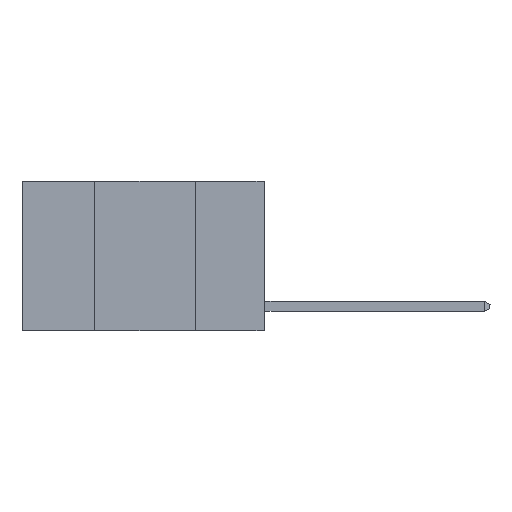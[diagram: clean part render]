
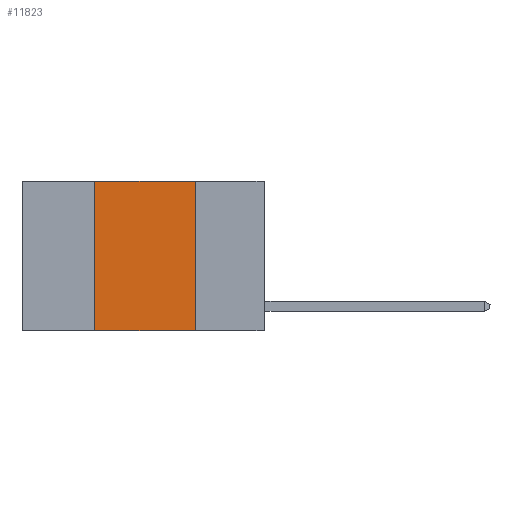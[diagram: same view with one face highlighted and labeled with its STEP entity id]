
A CAD part, left-side view. The second image highlights one B-rep face of the part: STEP entity #11823.
In plain terms, the highlighted planar face has unit normal (-1, 0, 0).
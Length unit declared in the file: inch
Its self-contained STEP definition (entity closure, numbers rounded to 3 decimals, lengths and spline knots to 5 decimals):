
#327 = VECTOR ( 'NONE', #13851, 39.37008 ) ;
#331 = CARTESIAN_POINT ( 'NONE',  ( 0., 0.6, 0. ) ) ;
#853 = LINE ( 'NONE', #331, #14843 ) ;
#2307 = VERTEX_POINT ( 'NONE', #4782 ) ;
#2994 = VERTEX_POINT ( 'NONE', #6998 ) ;
#4344 = CARTESIAN_POINT ( 'NONE',  ( 0., 0.42, 0. ) ) ;
#4782 = CARTESIAN_POINT ( 'NONE',  ( 0., 0.17, -0.37 ) ) ;
#4846 = EDGE_LOOP ( 'NONE', ( #9016, #16720, #15301, #22630 ) ) ;
#5851 = DIRECTION ( 'NONE',  ( 0., -1., 0. ) ) ;
#6039 = LINE ( 'NONE', #4344, #15748 ) ;
#6593 = CARTESIAN_POINT ( 'NONE',  ( 0., 0.6, -0.37 ) ) ;
#6890 = DIRECTION ( 'NONE',  ( 0., 0., -1. ) ) ;
#6998 = CARTESIAN_POINT ( 'NONE',  ( 0., 0.17, 0. ) ) ;
#7454 = CARTESIAN_POINT ( 'NONE',  ( 0., 0.6, 0. ) ) ;
#8240 = CARTESIAN_POINT ( 'NONE',  ( 0., 0.42, -0.37 ) ) ;
#8702 = CARTESIAN_POINT ( 'NONE',  ( 0., 0.17, 0. ) ) ;
#9016 = ORIENTED_EDGE ( 'NONE', *, *, #10426, .F. ) ;
#9424 = EDGE_CURVE ( 'NONE', #10244, #22296, #6039, .T. ) ;
#10043 = LINE ( 'NONE', #6593, #327 ) ;
#10093 = EDGE_CURVE ( 'NONE', #22296, #2994, #853, .T. ) ;
#10244 = VERTEX_POINT ( 'NONE', #8240 ) ;
#10426 = EDGE_CURVE ( 'NONE', #2994, #2307, #17103, .T. ) ;
#11143 = DIRECTION ( 'NONE',  ( 0., 0., -1. ) ) ;
#11823 = ADVANCED_FACE ( 'NONE', ( #20702 ), #12908, .F. ) ;
#12282 = VECTOR ( 'NONE', #6890, 39.37008 ) ;
#12908 = PLANE ( 'NONE',  #17434 ) ;
#12997 = CARTESIAN_POINT ( 'NONE',  ( 0., 0.42, 0. ) ) ;
#13851 = DIRECTION ( 'NONE',  ( 0., -1., 0. ) ) ;
#14843 = VECTOR ( 'NONE', #5851, 39.37008 ) ;
#15270 = DIRECTION ( 'NONE',  ( 0., 0., 1. ) ) ;
#15301 = ORIENTED_EDGE ( 'NONE', *, *, #9424, .F. ) ;
#15748 = VECTOR ( 'NONE', #15270, 39.37008 ) ;
#16720 = ORIENTED_EDGE ( 'NONE', *, *, #10093, .F. ) ;
#17103 = LINE ( 'NONE', #8702, #12282 ) ;
#17434 = AXIS2_PLACEMENT_3D ( 'NONE', #7454, #21950, #11143 ) ;
#19960 = EDGE_CURVE ( 'NONE', #10244, #2307, #10043, .T. ) ;
#20702 = FACE_OUTER_BOUND ( 'NONE', #4846, .T. ) ;
#21950 = DIRECTION ( 'NONE',  ( 1., 0., 0. ) ) ;
#22296 = VERTEX_POINT ( 'NONE', #12997 ) ;
#22630 = ORIENTED_EDGE ( 'NONE', *, *, #19960, .T. ) ;
